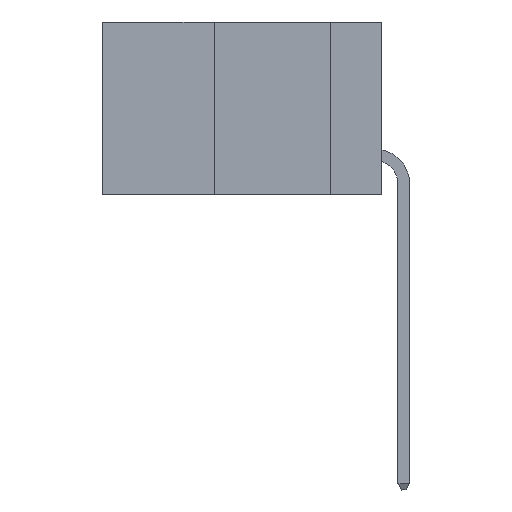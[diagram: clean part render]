
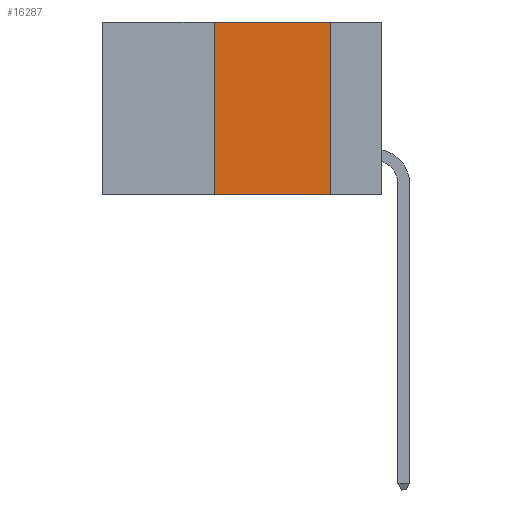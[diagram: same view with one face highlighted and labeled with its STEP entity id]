
A CAD part, left-side view. The second image highlights one B-rep face of the part: STEP entity #16287.
In plain terms, the highlighted planar face has unit normal (-1, 0, 0).
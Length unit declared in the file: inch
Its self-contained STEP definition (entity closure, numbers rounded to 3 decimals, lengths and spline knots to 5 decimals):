
#783 = EDGE_CURVE ( 'NONE', #26198, #29084, #16526, .T. ) ;
#838 = CARTESIAN_POINT ( 'NONE',  ( 0., 0.6, 0. ) ) ;
#1421 = AXIS2_PLACEMENT_3D ( 'NONE', #838, #29557, #15366 ) ;
#3189 = PLANE ( 'NONE',  #1421 ) ;
#4902 = LINE ( 'NONE', #12946, #15685 ) ;
#4926 = DIRECTION ( 'NONE',  ( 0., 0., -1. ) ) ;
#5639 = ORIENTED_EDGE ( 'NONE', *, *, #24613, .F. ) ;
#6843 = EDGE_CURVE ( 'NONE', #13200, #29953, #27333, .T. ) ;
#7153 = LINE ( 'NONE', #25706, #17498 ) ;
#8597 = DIRECTION ( 'NONE',  ( 0., -1., 0. ) ) ;
#9159 = CARTESIAN_POINT ( 'NONE',  ( 0., 0.11, 0. ) ) ;
#10189 = EDGE_CURVE ( 'NONE', #26198, #29953, #4902, .T. ) ;
#11560 = DIRECTION ( 'NONE',  ( 0., -1., 0. ) ) ;
#12946 = CARTESIAN_POINT ( 'NONE',  ( 0., 0.6, -0.37 ) ) ;
#13200 = VERTEX_POINT ( 'NONE', #15288 ) ;
#13788 = CARTESIAN_POINT ( 'NONE',  ( 0., 0.11, -0.37 ) ) ;
#15288 = CARTESIAN_POINT ( 'NONE',  ( 0., 0.11, 0. ) ) ;
#15315 = ORIENTED_EDGE ( 'NONE', *, *, #10189, .T. ) ;
#15366 = DIRECTION ( 'NONE',  ( 0., 0., -1. ) ) ;
#15685 = VECTOR ( 'NONE', #8597, 39.37008 ) ;
#16096 = EDGE_LOOP ( 'NONE', ( #26539, #5639, #22034, #15315 ) ) ;
#16287 = ADVANCED_FACE ( 'NONE', ( #17213 ), #3189, .F. ) ;
#16526 = LINE ( 'NONE', #20362, #29140 ) ;
#17213 = FACE_OUTER_BOUND ( 'NONE', #16096, .T. ) ;
#17498 = VECTOR ( 'NONE', #11560, 39.37008 ) ;
#20362 = CARTESIAN_POINT ( 'NONE',  ( 0., 0.36, 0. ) ) ;
#22034 = ORIENTED_EDGE ( 'NONE', *, *, #783, .F. ) ;
#24613 = EDGE_CURVE ( 'NONE', #29084, #13200, #7153, .T. ) ;
#24714 = CARTESIAN_POINT ( 'NONE',  ( 0., 0.36, 0. ) ) ;
#25706 = CARTESIAN_POINT ( 'NONE',  ( 0., 0.6, 0. ) ) ;
#26198 = VERTEX_POINT ( 'NONE', #29959 ) ;
#26539 = ORIENTED_EDGE ( 'NONE', *, *, #6843, .F. ) ;
#27333 = LINE ( 'NONE', #9159, #29952 ) ;
#29084 = VERTEX_POINT ( 'NONE', #24714 ) ;
#29140 = VECTOR ( 'NONE', #29729, 39.37008 ) ;
#29557 = DIRECTION ( 'NONE',  ( 1., 0., 0. ) ) ;
#29729 = DIRECTION ( 'NONE',  ( 0., 0., 1. ) ) ;
#29952 = VECTOR ( 'NONE', #4926, 39.37008 ) ;
#29953 = VERTEX_POINT ( 'NONE', #13788 ) ;
#29959 = CARTESIAN_POINT ( 'NONE',  ( 0., 0.36, -0.37 ) ) ;
